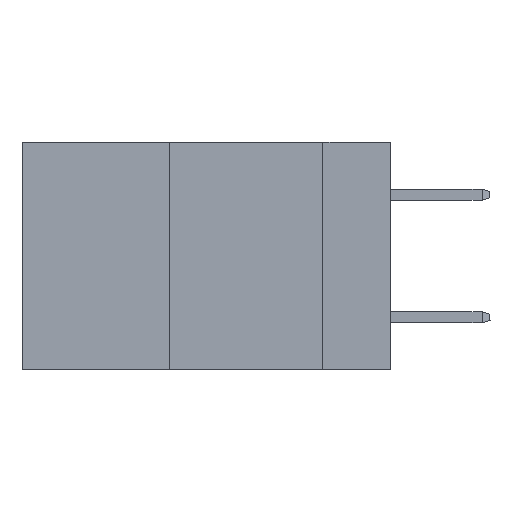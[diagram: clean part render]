
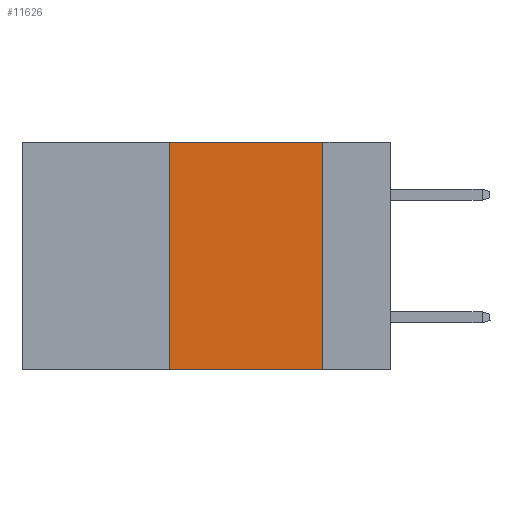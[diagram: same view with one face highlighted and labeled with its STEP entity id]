
A CAD part, left-side view. The second image highlights one B-rep face of the part: STEP entity #11626.
In plain terms, the highlighted planar face has unit normal (-1, 0, 0).
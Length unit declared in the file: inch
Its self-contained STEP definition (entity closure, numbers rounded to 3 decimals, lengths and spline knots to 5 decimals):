
#289 = VECTOR ( 'NONE', #17943, 39.37008 ) ;
#6015 = EDGE_CURVE ( 'NONE', #24417, #15222, #30416, .T. ) ;
#7979 = ORIENTED_EDGE ( 'NONE', *, *, #17554, .T. ) ;
#8577 = DIRECTION ( 'NONE',  ( 1., 0., 0. ) ) ;
#10973 = DIRECTION ( 'NONE',  ( 0., -1., 0. ) ) ;
#11056 = CARTESIAN_POINT ( 'NONE',  ( 0., 0.6, 0. ) ) ;
#11626 = ADVANCED_FACE ( 'NONE', ( #37225 ), #31372, .F. ) ;
#12184 = CARTESIAN_POINT ( 'NONE',  ( 0., 0.6, -0.37 ) ) ;
#12698 = ORIENTED_EDGE ( 'NONE', *, *, #6015, .F. ) ;
#13916 = AXIS2_PLACEMENT_3D ( 'NONE', #11056, #8577, #17330 ) ;
#13992 = EDGE_LOOP ( 'NONE', ( #26366, #37382, #12698, #7979 ) ) ;
#14517 = CARTESIAN_POINT ( 'NONE',  ( 0., 0.11, 0. ) ) ;
#15222 = VERTEX_POINT ( 'NONE', #30033 ) ;
#16500 = CARTESIAN_POINT ( 'NONE',  ( 0., 0.6, 0. ) ) ;
#16689 = LINE ( 'NONE', #16500, #32768 ) ;
#16771 = CARTESIAN_POINT ( 'NONE',  ( 0., 0.11, 0. ) ) ;
#17330 = DIRECTION ( 'NONE',  ( 0., 0., -1. ) ) ;
#17554 = EDGE_CURVE ( 'NONE', #24417, #30381, #34970, .T. ) ;
#17943 = DIRECTION ( 'NONE',  ( 0., 0., -1. ) ) ;
#21513 = CARTESIAN_POINT ( 'NONE',  ( 0., 0.36, 0. ) ) ;
#23970 = DIRECTION ( 'NONE',  ( 0., 0., 1. ) ) ;
#24417 = VERTEX_POINT ( 'NONE', #24505 ) ;
#24505 = CARTESIAN_POINT ( 'NONE',  ( 0., 0.36, -0.37 ) ) ;
#24879 = VECTOR ( 'NONE', #28931, 39.37008 ) ;
#26366 = ORIENTED_EDGE ( 'NONE', *, *, #29882, .F. ) ;
#27805 = VERTEX_POINT ( 'NONE', #16771 ) ;
#28931 = DIRECTION ( 'NONE',  ( 0., -1., 0. ) ) ;
#29882 = EDGE_CURVE ( 'NONE', #27805, #30381, #35384, .T. ) ;
#30033 = CARTESIAN_POINT ( 'NONE',  ( 0., 0.36, 0. ) ) ;
#30381 = VERTEX_POINT ( 'NONE', #32494 ) ;
#30416 = LINE ( 'NONE', #21513, #36686 ) ;
#31372 = PLANE ( 'NONE',  #13916 ) ;
#32494 = CARTESIAN_POINT ( 'NONE',  ( 0., 0.11, -0.37 ) ) ;
#32768 = VECTOR ( 'NONE', #10973, 39.37008 ) ;
#34970 = LINE ( 'NONE', #12184, #24879 ) ;
#35384 = LINE ( 'NONE', #14517, #289 ) ;
#36686 = VECTOR ( 'NONE', #23970, 39.37008 ) ;
#37225 = FACE_OUTER_BOUND ( 'NONE', #13992, .T. ) ;
#37382 = ORIENTED_EDGE ( 'NONE', *, *, #37428, .F. ) ;
#37428 = EDGE_CURVE ( 'NONE', #15222, #27805, #16689, .T. ) ;
